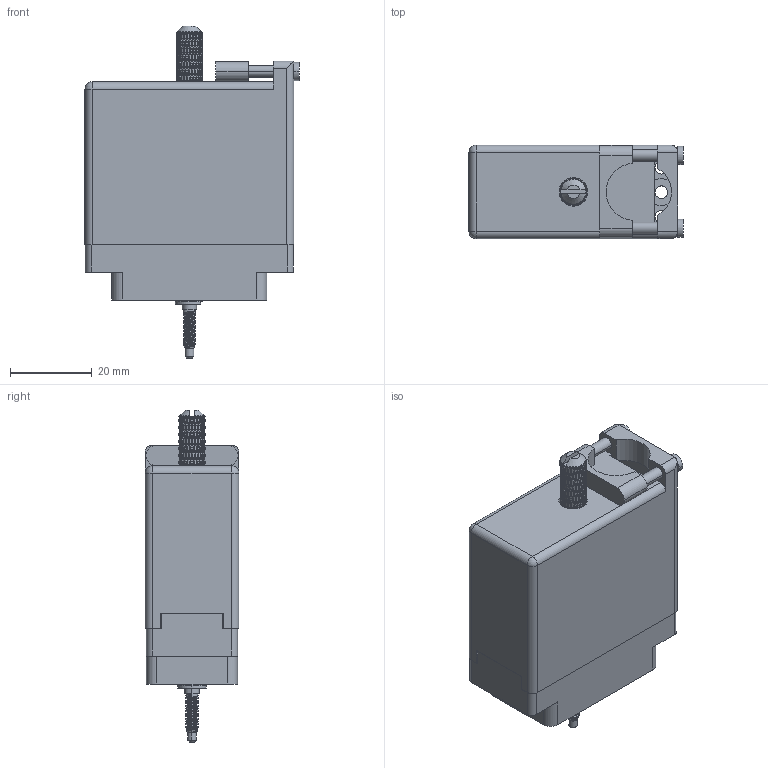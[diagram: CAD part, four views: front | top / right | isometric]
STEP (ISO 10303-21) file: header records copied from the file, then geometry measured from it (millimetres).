
FILE_DESCRIPTION (( 'STEP AP203' ), '1' );
FILE_NAME ('519-036-000-365.STEP', '2020-03-02T21:40:53', ( '' ), ( '' ), 'SwSTEP 2.0', 'SolidWorks 2016', '' );
FILE_SCHEMA (( 'CONFIG_CONTROL_DESIGN' ));
Length unit declared in the file: inch
Products named in the file (8): 516-251-035-100; 516-253-035-100; 519 Plug Insulator_036; 519-036-000-365; 516-230-001_Metal - 038 Top Entry; Actuating Screw Assy 038-056; 516-250-038-111; 516-253-138-107
Assembly tree (8 placements, depth 3):
  519-036-000-365
    519 Plug Insulator_036
    Actuating Screw Assy 038-056
      516-251-035-100
      516-253-035-100  x2
      516-253-138-107
      516-250-038-111
    516-230-001_Metal - 038 Top Entry
Bounding box: 52.27 x 22.83 x 81.03 mm (x, y, z)
Volume: 19988.9 mm3; surface area: 27478.7 mm2
Topology: 7 solids, 7 shells, 2318 faces, 5683 edges, 3396 vertices
Faces by surface type: bspline 1006, plane 724, cylinder 566, cone 20, sphere 2
Entity records: 97704 total; most frequent: CARTESIAN_POINT 53586, ORIENTED_EDGE 11338, DIRECTION 6500, EDGE_CURVE 5669, VERTEX_POINT 3388, EDGE_LOOP 2431, ADVANCED_FACE 2312, FACE_OUTER_BOUND 2312
